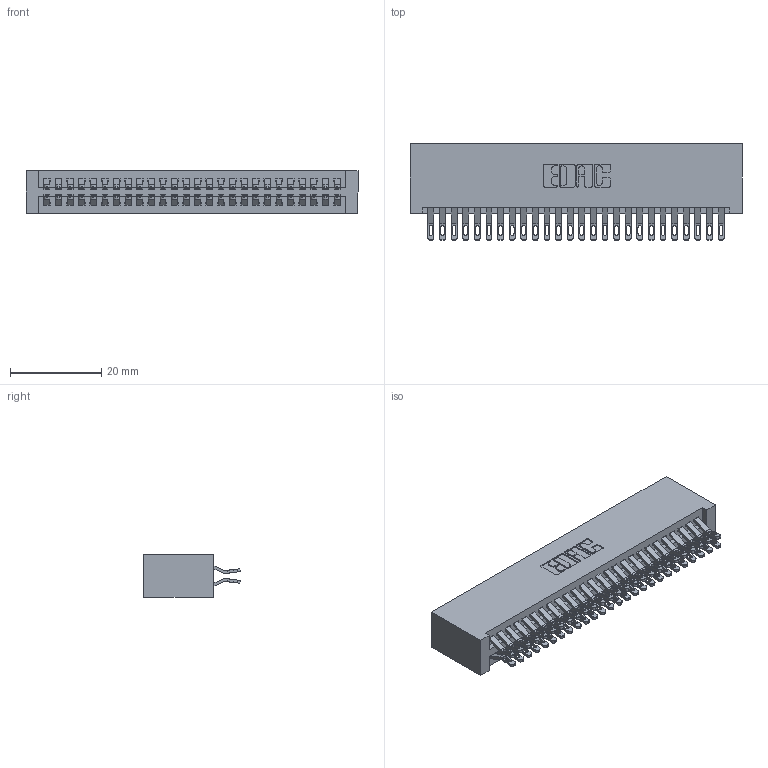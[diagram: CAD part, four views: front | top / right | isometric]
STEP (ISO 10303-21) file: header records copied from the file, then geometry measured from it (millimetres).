
FILE_DESCRIPTION (( 'STEP AP203' ), '1' );
FILE_NAME ('345-052-555-201.STEP', '2019-10-29T17:04:19', ( '' ), ( '' ), 'SwSTEP 2.0', 'SolidWorks 2016', '' );
FILE_SCHEMA (( 'CONFIG_CONTROL_DESIGN' ));
Length unit declared in the file: inch
Products named in the file (3): 345-292-001_555 Tail; 345-052-555-201; 345 Part_No Mounting Lugs
Assembly tree (53 placements, depth 2):
  345-052-555-201
    345 Part_No Mounting Lugs
    345-292-001_555 Tail  x52
Bounding box: 72.64 x 21.13 x 9.4 mm (x, y, z)
Volume: 7674.9 mm3; surface area: 11862.8 mm2
Topology: 53 solids, 53 shells, 3030 faces, 9521 edges, 6346 vertices
Faces by surface type: plane 1688, cylinder 1342
Entity records: 22603 total; most frequent: CARTESIAN_POINT 3838, ORIENTED_EDGE 3742, DIRECTION 3367, EDGE_CURVE 1871, LINE 1623, VECTOR 1623, VERTEX_POINT 1246, AXIS2_PLACEMENT_3D 872
